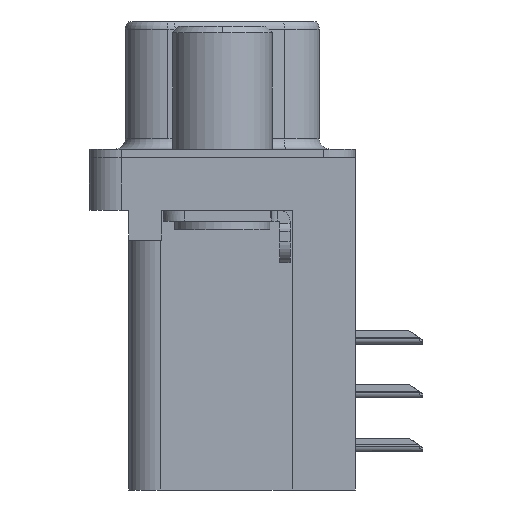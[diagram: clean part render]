
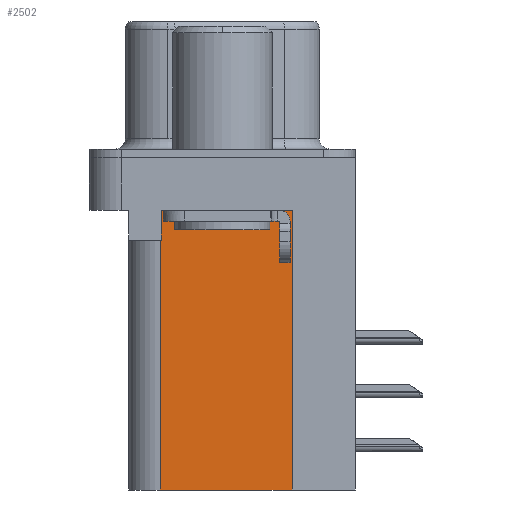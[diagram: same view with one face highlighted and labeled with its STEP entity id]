
A CAD part, left-side view. The second image highlights one B-rep face of the part: STEP entity #2502.
In plain terms, the highlighted planar face has unit normal (-1, 0, 0).
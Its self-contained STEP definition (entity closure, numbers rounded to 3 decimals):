
#64 = DIRECTION ( 'NONE',  ( 1., 0., 0. ) ) ;
#547 = CARTESIAN_POINT ( 'NONE',  ( 3.7, -3.295, -15.7 ) ) ;
#884 = LINE ( 'NONE', #20880, #5555 ) ;
#1022 = VERTEX_POINT ( 'NONE', #19725 ) ;
#1024 = EDGE_CURVE ( 'NONE', #8838, #8098, #29107, .T. ) ;
#1429 = EDGE_CURVE ( 'NONE', #8098, #10114, #9532, .T. ) ;
#2145 = ORIENTED_EDGE ( 'NONE', *, *, #1429, .F. ) ;
#2502 = ADVANCED_FACE ( 'NONE', ( #8103 ), #16575, .F. ) ;
#3782 = CARTESIAN_POINT ( 'NONE',  ( 3.7, -3.295, -15.7 ) ) ;
#4211 = CARTESIAN_POINT ( 'NONE',  ( 3.7, 2.895, -3.9 ) ) ;
#4275 = DIRECTION ( 'NONE',  ( 0., 0., 1. ) ) ;
#4617 = DIRECTION ( 'NONE',  ( 0., 1., 0. ) ) ;
#5555 = VECTOR ( 'NONE', #25432, 1000. ) ;
#5608 = EDGE_CURVE ( 'NONE', #1022, #18077, #28966, .T. ) ;
#5626 = ORIENTED_EDGE ( 'NONE', *, *, #5608, .T. ) ;
#5691 = VECTOR ( 'NONE', #20254, 1000. ) ;
#6568 = CARTESIAN_POINT ( 'NONE',  ( 3.7, 2.895, -2.5 ) ) ;
#6941 = ORIENTED_EDGE ( 'NONE', *, *, #14732, .T. ) ;
#8098 = VERTEX_POINT ( 'NONE', #25789 ) ;
#8103 = FACE_OUTER_BOUND ( 'NONE', #22824, .T. ) ;
#8838 = VERTEX_POINT ( 'NONE', #3782 ) ;
#9532 = LINE ( 'NONE', #20319, #14873 ) ;
#10114 = VERTEX_POINT ( 'NONE', #19951 ) ;
#10762 = CARTESIAN_POINT ( 'NONE',  ( 3.7, 0., -3.9 ) ) ;
#11050 = LINE ( 'NONE', #4211, #5691 ) ;
#11246 = DIRECTION ( 'NONE',  ( 0., 1., 0. ) ) ;
#12937 = ORIENTED_EDGE ( 'NONE', *, *, #14950, .T. ) ;
#13557 = CARTESIAN_POINT ( 'NONE',  ( 3.7, -3.295, -2.5 ) ) ;
#13912 = ORIENTED_EDGE ( 'NONE', *, *, #19018, .T. ) ;
#14732 = EDGE_CURVE ( 'NONE', #16894, #10114, #16060, .T. ) ;
#14873 = VECTOR ( 'NONE', #4275, 1000. ) ;
#14950 = EDGE_CURVE ( 'NONE', #18077, #16894, #11050, .T. ) ;
#15339 = DIRECTION ( 'NONE',  ( 0., 1., 0. ) ) ;
#16060 = LINE ( 'NONE', #10762, #27474 ) ;
#16515 = DIRECTION ( 'NONE',  ( 0., 0., -1. ) ) ;
#16575 = PLANE ( 'NONE',  #16614 ) ;
#16614 = AXIS2_PLACEMENT_3D ( 'NONE', #16679, #64, #16515 ) ;
#16679 = CARTESIAN_POINT ( 'NONE',  ( 3.7, -3.295, -15.7 ) ) ;
#16894 = VERTEX_POINT ( 'NONE', #27466 ) ;
#18077 = VERTEX_POINT ( 'NONE', #6568 ) ;
#19018 = EDGE_CURVE ( 'NONE', #8838, #1022, #884, .T. ) ;
#19725 = CARTESIAN_POINT ( 'NONE',  ( 3.7, -3.295, -2.5 ) ) ;
#19951 = CARTESIAN_POINT ( 'NONE',  ( 3.7, 2.925, -3.9 ) ) ;
#20254 = DIRECTION ( 'NONE',  ( 0., 0., -1. ) ) ;
#20319 = CARTESIAN_POINT ( 'NONE',  ( 3.7, 2.925, -15.7 ) ) ;
#20880 = CARTESIAN_POINT ( 'NONE',  ( 3.7, -3.295, -15.7 ) ) ;
#22704 = ORIENTED_EDGE ( 'NONE', *, *, #1024, .F. ) ;
#22824 = EDGE_LOOP ( 'NONE', ( #5626, #12937, #6941, #2145, #22704, #13912 ) ) ;
#23084 = VECTOR ( 'NONE', #4617, 1000. ) ;
#25432 = DIRECTION ( 'NONE',  ( 0., 0., 1. ) ) ;
#25789 = CARTESIAN_POINT ( 'NONE',  ( 3.7, 2.925, -15.7 ) ) ;
#27466 = CARTESIAN_POINT ( 'NONE',  ( 3.7, 2.895, -3.9 ) ) ;
#27474 = VECTOR ( 'NONE', #15339, 1000. ) ;
#28249 = VECTOR ( 'NONE', #11246, 1000. ) ;
#28966 = LINE ( 'NONE', #13557, #28249 ) ;
#29107 = LINE ( 'NONE', #547, #23084 ) ;
